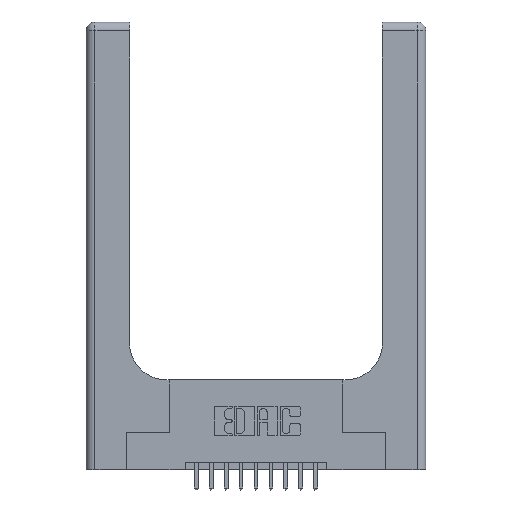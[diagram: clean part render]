
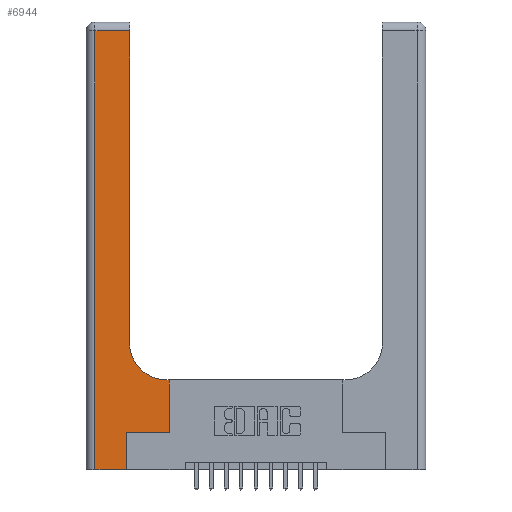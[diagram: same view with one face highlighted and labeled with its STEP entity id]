
A CAD part, top view. The second image highlights one B-rep face of the part: STEP entity #6944.
In plain terms, the highlighted planar face has unit normal (0, 0, 1).
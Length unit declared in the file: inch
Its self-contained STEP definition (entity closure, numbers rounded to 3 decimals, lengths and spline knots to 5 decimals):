
#294 = ORIENTED_EDGE ( 'NONE', *, *, #4102, .T. ) ;
#330 = CARTESIAN_POINT ( 'NONE',  ( 0.5415, 0.85, 0.37 ) ) ;
#514 = ORIENTED_EDGE ( 'NONE', *, *, #5511, .T. ) ;
#533 = DIRECTION ( 'NONE',  ( 0., 1., 0. ) ) ;
#618 = ORIENTED_EDGE ( 'NONE', *, *, #9952, .T. ) ;
#834 = VECTOR ( 'NONE', #14590, 39.37008 ) ;
#855 = CARTESIAN_POINT ( 'NONE',  ( 0.269, 0., 0.37 ) ) ;
#920 = EDGE_CURVE ( 'NONE', #14951, #3945, #12074, .T. ) ;
#1474 = CARTESIAN_POINT ( 'NONE',  ( 0.5585, 0.25, 0.37 ) ) ;
#1569 = DIRECTION ( 'NONE',  ( 0., 0., -1. ) ) ;
#1650 = EDGE_CURVE ( 'NONE', #12829, #14951, #7416, .T. ) ;
#1706 = ORIENTED_EDGE ( 'NONE', *, *, #10920, .T. ) ;
#1830 = CARTESIAN_POINT ( 'NONE',  ( 0.269, 0., 0.37 ) ) ;
#1905 = VERTEX_POINT ( 'NONE', #10520 ) ;
#1976 = VECTOR ( 'NONE', #6242, 39.37008 ) ;
#2167 = DIRECTION ( 'NONE',  ( -1., 0., 0. ) ) ;
#2485 = CARTESIAN_POINT ( 'NONE',  ( 0., 3., 0.37 ) ) ;
#3163 = AXIS2_PLACEMENT_3D ( 'NONE', #2485, #14068, #16697 ) ;
#3294 = CARTESIAN_POINT ( 'NONE',  ( 0.2915, 0.85, 0.37 ) ) ;
#3416 = VECTOR ( 'NONE', #10916, 39.37008 ) ;
#3420 = CARTESIAN_POINT ( 'NONE',  ( 0.2915, 0.6, 0.37 ) ) ;
#3486 = ORIENTED_EDGE ( 'NONE', *, *, #16353, .T. ) ;
#3816 = VECTOR ( 'NONE', #6737, 39.37008 ) ;
#3945 = VERTEX_POINT ( 'NONE', #1830 ) ;
#4102 = EDGE_CURVE ( 'NONE', #14167, #10537, #4647, .T. ) ;
#4170 = CARTESIAN_POINT ( 'NONE',  ( 0.269, 0.25, 0.37 ) ) ;
#4204 = CARTESIAN_POINT ( 'NONE',  ( 0., 0., 0.37 ) ) ;
#4435 = CARTESIAN_POINT ( 'NONE',  ( 0., 2.94, 0.37 ) ) ;
#4647 = LINE ( 'NONE', #1474, #6861 ) ;
#5013 = CARTESIAN_POINT ( 'NONE',  ( 0.269, 0.25, 0.37 ) ) ;
#5187 = LINE ( 'NONE', #4170, #3816 ) ;
#5446 = LINE ( 'NONE', #855, #834 ) ;
#5511 = EDGE_CURVE ( 'NONE', #11710, #14034, #13098, .T. ) ;
#5636 = DIRECTION ( 'NONE',  ( 0., 1., 0. ) ) ;
#6242 = DIRECTION ( 'NONE',  ( 0., -1., 0. ) ) ;
#6389 = PLANE ( 'NONE',  #3163 ) ;
#6624 = VECTOR ( 'NONE', #2167, 39.37008 ) ;
#6672 = VERTEX_POINT ( 'NONE', #5013 ) ;
#6737 = DIRECTION ( 'NONE',  ( 1., 0., 0. ) ) ;
#6775 = DIRECTION ( 'NONE',  ( 1., 0., 0. ) ) ;
#6861 = VECTOR ( 'NONE', #5636, 39.37008 ) ;
#6944 = ADVANCED_FACE ( 'NONE', ( #15858 ), #6389, .F. ) ;
#7416 = LINE ( 'NONE', #7865, #1976 ) ;
#7865 = CARTESIAN_POINT ( 'NONE',  ( 0.06, 3., 0.37 ) ) ;
#8107 = ORIENTED_EDGE ( 'NONE', *, *, #920, .T. ) ;
#8224 = AXIS2_PLACEMENT_3D ( 'NONE', #330, #1569, #11760 ) ;
#8569 = CARTESIAN_POINT ( 'NONE',  ( 0.06, 0., 0.37 ) ) ;
#9010 = VECTOR ( 'NONE', #533, 39.37008 ) ;
#9321 = CARTESIAN_POINT ( 'NONE',  ( 0.5585, 0.6, 0.37 ) ) ;
#9597 = LINE ( 'NONE', #12214, #9010 ) ;
#9952 = EDGE_CURVE ( 'NONE', #6672, #14167, #5187, .T. ) ;
#10039 = LINE ( 'NONE', #3420, #6624 ) ;
#10520 = CARTESIAN_POINT ( 'NONE',  ( 0.2915, 2.94, 0.37 ) ) ;
#10537 = VERTEX_POINT ( 'NONE', #9321 ) ;
#10916 = DIRECTION ( 'NONE',  ( -1., 0., 0. ) ) ;
#10920 = EDGE_CURVE ( 'NONE', #1905, #12829, #13668, .T. ) ;
#11375 = EDGE_CURVE ( 'NONE', #14034, #1905, #9597, .T. ) ;
#11710 = VERTEX_POINT ( 'NONE', #13656 ) ;
#11760 = DIRECTION ( 'NONE',  ( 1., 0., 0. ) ) ;
#11830 = ORIENTED_EDGE ( 'NONE', *, *, #14954, .T. ) ;
#11903 = ORIENTED_EDGE ( 'NONE', *, *, #1650, .T. ) ;
#12007 = CARTESIAN_POINT ( 'NONE',  ( 0.06, 2.94, 0.37 ) ) ;
#12074 = LINE ( 'NONE', #4204, #14680 ) ;
#12214 = CARTESIAN_POINT ( 'NONE',  ( 0.2915, 3., 0.37 ) ) ;
#12739 = CARTESIAN_POINT ( 'NONE',  ( 0.5585, 0.25, 0.37 ) ) ;
#12829 = VERTEX_POINT ( 'NONE', #12007 ) ;
#13098 = CIRCLE ( 'NONE', #8224, 0.25 ) ;
#13199 = EDGE_LOOP ( 'NONE', ( #14854, #1706, #11903, #8107, #11830, #618, #294, #3486, #514 ) ) ;
#13656 = CARTESIAN_POINT ( 'NONE',  ( 0.5415, 0.6, 0.37 ) ) ;
#13668 = LINE ( 'NONE', #4435, #3416 ) ;
#14034 = VERTEX_POINT ( 'NONE', #3294 ) ;
#14068 = DIRECTION ( 'NONE',  ( 0., 0., -1. ) ) ;
#14167 = VERTEX_POINT ( 'NONE', #12739 ) ;
#14590 = DIRECTION ( 'NONE',  ( 0., 1., 0. ) ) ;
#14680 = VECTOR ( 'NONE', #6775, 39.37008 ) ;
#14854 = ORIENTED_EDGE ( 'NONE', *, *, #11375, .T. ) ;
#14951 = VERTEX_POINT ( 'NONE', #8569 ) ;
#14954 = EDGE_CURVE ( 'NONE', #3945, #6672, #5446, .T. ) ;
#15858 = FACE_OUTER_BOUND ( 'NONE', #13199, .T. ) ;
#16353 = EDGE_CURVE ( 'NONE', #10537, #11710, #10039, .T. ) ;
#16697 = DIRECTION ( 'NONE',  ( -1., 0., 0. ) ) ;
